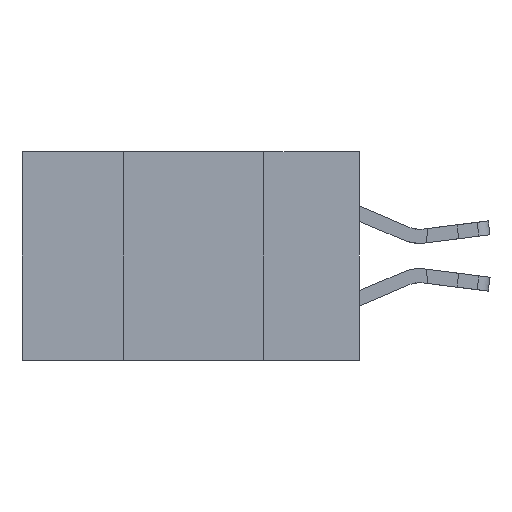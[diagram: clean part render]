
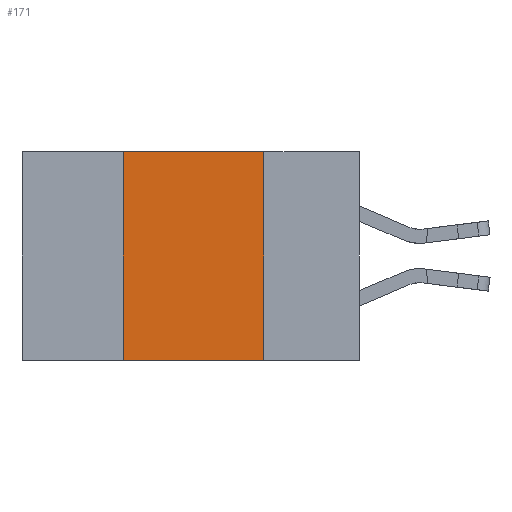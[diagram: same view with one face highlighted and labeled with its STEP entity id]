
A CAD part, left-side view. The second image highlights one B-rep face of the part: STEP entity #171.
In plain terms, the highlighted planar face has unit normal (-1, 0, 0).
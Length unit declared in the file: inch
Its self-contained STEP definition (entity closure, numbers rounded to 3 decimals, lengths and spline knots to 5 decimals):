
#171 = ADVANCED_FACE ( 'NONE', ( #24703 ), #4144, .F. ) ;
#227 = LINE ( 'NONE', #6127, #8903 ) ;
#946 = ORIENTED_EDGE ( 'NONE', *, *, #28382, .F. ) ;
#1152 = CARTESIAN_POINT ( 'NONE',  ( 0., 0.6, 0. ) ) ;
#1495 = VERTEX_POINT ( 'NONE', #4001 ) ;
#1499 = DIRECTION ( 'NONE',  ( 0., 0., -1. ) ) ;
#1816 = EDGE_CURVE ( 'NONE', #1495, #21580, #21319, .T. ) ;
#2227 = ORIENTED_EDGE ( 'NONE', *, *, #1816, .T. ) ;
#3206 = VECTOR ( 'NONE', #32389, 39.37008 ) ;
#3554 = LINE ( 'NONE', #31165, #22892 ) ;
#4001 = CARTESIAN_POINT ( 'NONE',  ( 0., 0.42, -0.37 ) ) ;
#4144 = PLANE ( 'NONE',  #33383 ) ;
#5917 = DIRECTION ( 'NONE',  ( 0., -1., 0. ) ) ;
#6127 = CARTESIAN_POINT ( 'NONE',  ( 0., 0.6, 0. ) ) ;
#7683 = VERTEX_POINT ( 'NONE', #30383 ) ;
#8903 = VECTOR ( 'NONE', #5917, 39.37008 ) ;
#9601 = CARTESIAN_POINT ( 'NONE',  ( 0., 0.42, 0. ) ) ;
#11004 = VECTOR ( 'NONE', #12733, 39.37008 ) ;
#11805 = EDGE_CURVE ( 'NONE', #1495, #18846, #3554, .T. ) ;
#12733 = DIRECTION ( 'NONE',  ( 0., -1., 0. ) ) ;
#18505 = CARTESIAN_POINT ( 'NONE',  ( 0., 0.6, -0.37 ) ) ;
#18846 = VERTEX_POINT ( 'NONE', #9601 ) ;
#21319 = LINE ( 'NONE', #18505, #11004 ) ;
#21580 = VERTEX_POINT ( 'NONE', #33861 ) ;
#22892 = VECTOR ( 'NONE', #25521, 39.37008 ) ;
#24703 = FACE_OUTER_BOUND ( 'NONE', #31066, .T. ) ;
#24996 = LINE ( 'NONE', #26512, #3206 ) ;
#25521 = DIRECTION ( 'NONE',  ( 0., 0., 1. ) ) ;
#26512 = CARTESIAN_POINT ( 'NONE',  ( 0., 0.17, 0. ) ) ;
#27560 = DIRECTION ( 'NONE',  ( 1., 0., 0. ) ) ;
#28220 = ORIENTED_EDGE ( 'NONE', *, *, #32404, .F. ) ;
#28382 = EDGE_CURVE ( 'NONE', #7683, #21580, #24996, .T. ) ;
#30383 = CARTESIAN_POINT ( 'NONE',  ( 0., 0.17, 0. ) ) ;
#31066 = EDGE_LOOP ( 'NONE', ( #946, #28220, #32372, #2227 ) ) ;
#31165 = CARTESIAN_POINT ( 'NONE',  ( 0., 0.42, 0. ) ) ;
#32372 = ORIENTED_EDGE ( 'NONE', *, *, #11805, .F. ) ;
#32389 = DIRECTION ( 'NONE',  ( 0., 0., -1. ) ) ;
#32404 = EDGE_CURVE ( 'NONE', #18846, #7683, #227, .T. ) ;
#33383 = AXIS2_PLACEMENT_3D ( 'NONE', #1152, #27560, #1499 ) ;
#33861 = CARTESIAN_POINT ( 'NONE',  ( 0., 0.17, -0.37 ) ) ;
